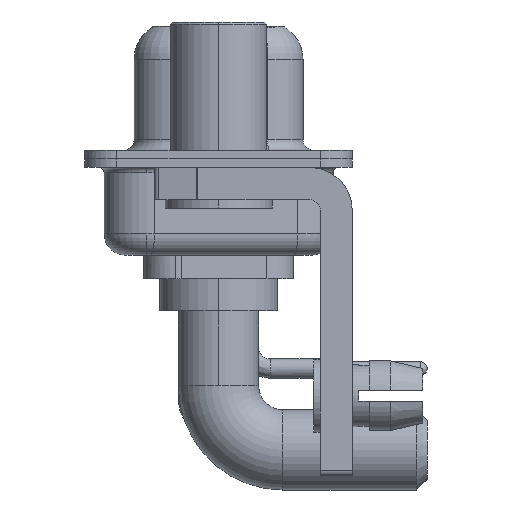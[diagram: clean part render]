
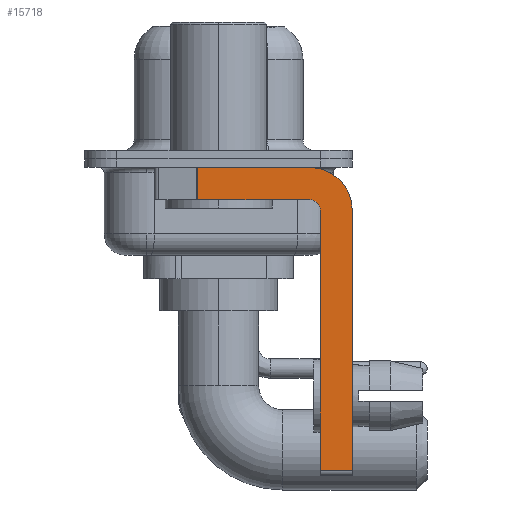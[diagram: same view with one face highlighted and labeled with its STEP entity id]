
A CAD part, left-side view. The second image highlights one B-rep face of the part: STEP entity #15718.
In plain terms, the highlighted planar face has unit normal (-1, 0, 0).
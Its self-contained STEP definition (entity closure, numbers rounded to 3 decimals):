
#17 = ORIENTED_EDGE ( 'NONE', *, *, #8436, .F. ) ;
#399 = CARTESIAN_POINT ( 'NONE',  ( -2.9, 0.978, -1.9 ) ) ;
#597 = VERTEX_POINT ( 'NONE', #4582 ) ;
#678 = EDGE_CURVE ( 'NONE', #4930, #9148, #13054, .T. ) ;
#1188 = CARTESIAN_POINT ( 'NONE',  ( -2.9, -4.75, -14.55 ) ) ;
#1609 = CARTESIAN_POINT ( 'NONE',  ( -2.9, -4.25, -1.9 ) ) ;
#1646 = CARTESIAN_POINT ( 'NONE',  ( -2.9, -4.25, -2.4 ) ) ;
#2113 = LINE ( 'NONE', #8440, #13359 ) ;
#2677 = CARTESIAN_POINT ( 'NONE',  ( -2.9, -4.75, -14.8 ) ) ;
#2889 = ORIENTED_EDGE ( 'NONE', *, *, #14092, .T. ) ;
#3079 = FACE_OUTER_BOUND ( 'NONE', #19467, .T. ) ;
#3131 = ORIENTED_EDGE ( 'NONE', *, *, #19340, .F. ) ;
#3288 = VERTEX_POINT ( 'NONE', #1609 ) ;
#3504 = EDGE_CURVE ( 'NONE', #13564, #3627, #6079, .T. ) ;
#3627 = VERTEX_POINT ( 'NONE', #12449 ) ;
#3746 = AXIS2_PLACEMENT_3D ( 'NONE', #14241, #12507, #4745 ) ;
#3774 = AXIS2_PLACEMENT_3D ( 'NONE', #7189, #13382, #18751 ) ;
#3878 = EDGE_CURVE ( 'NONE', #7032, #13564, #2113, .T. ) ;
#3907 = VERTEX_POINT ( 'NONE', #13589 ) ;
#4548 = PLANE ( 'NONE',  #3746 ) ;
#4582 = CARTESIAN_POINT ( 'NONE',  ( -2.9, -4.75, -2.4 ) ) ;
#4745 = DIRECTION ( 'NONE',  ( 0., 0., -1. ) ) ;
#4930 = VERTEX_POINT ( 'NONE', #1188 ) ;
#5859 = CARTESIAN_POINT ( 'NONE',  ( -2.9, -6.25, -14.55 ) ) ;
#6079 = CIRCLE ( 'NONE', #3774, 2. ) ;
#6417 = DIRECTION ( 'NONE',  ( -1., 0., 0. ) ) ;
#6892 = EDGE_CURVE ( 'NONE', #4930, #597, #10350, .T. ) ;
#7032 = VERTEX_POINT ( 'NONE', #11185 ) ;
#7189 = CARTESIAN_POINT ( 'NONE',  ( -2.9, -4.25, -2.4 ) ) ;
#7872 = EDGE_CURVE ( 'NONE', #3627, #9148, #12156, .T. ) ;
#8357 = LINE ( 'NONE', #399, #18548 ) ;
#8436 = EDGE_CURVE ( 'NONE', #597, #3288, #13116, .T. ) ;
#8440 = CARTESIAN_POINT ( 'NONE',  ( -2.9, 3., -0.4 ) ) ;
#9043 = ORIENTED_EDGE ( 'NONE', *, *, #3878, .F. ) ;
#9148 = VERTEX_POINT ( 'NONE', #5859 ) ;
#9483 = ORIENTED_EDGE ( 'NONE', *, *, #678, .T. ) ;
#10350 = LINE ( 'NONE', #2677, #20332 ) ;
#11185 = CARTESIAN_POINT ( 'NONE',  ( -2.9, 0.978, -0.4 ) ) ;
#11782 = VECTOR ( 'NONE', #18347, 1000. ) ;
#12050 = CARTESIAN_POINT ( 'NONE',  ( -2.9, -4.25, -1.9 ) ) ;
#12125 = AXIS2_PLACEMENT_3D ( 'NONE', #1646, #6417, #12823 ) ;
#12156 = LINE ( 'NONE', #17004, #11782 ) ;
#12449 = CARTESIAN_POINT ( 'NONE',  ( -2.9, -6.25, -2.4 ) ) ;
#12507 = DIRECTION ( 'NONE',  ( 1., 0., 0. ) ) ;
#12823 = DIRECTION ( 'NONE',  ( 0., 0., 1. ) ) ;
#13010 = DIRECTION ( 'NONE',  ( 0., 0., -1. ) ) ;
#13054 = LINE ( 'NONE', #17699, #19336 ) ;
#13116 = CIRCLE ( 'NONE', #12125, 0.5 ) ;
#13359 = VECTOR ( 'NONE', #19493, 1000. ) ;
#13382 = DIRECTION ( 'NONE',  ( 1., 0., 0. ) ) ;
#13564 = VERTEX_POINT ( 'NONE', #19137 ) ;
#13589 = CARTESIAN_POINT ( 'NONE',  ( -2.9, 0.978, -1.9 ) ) ;
#14092 = EDGE_CURVE ( 'NONE', #7032, #3907, #8357, .T. ) ;
#14241 = CARTESIAN_POINT ( 'NONE',  ( -2.9, -4.25, -2.4 ) ) ;
#15228 = ORIENTED_EDGE ( 'NONE', *, *, #6892, .F. ) ;
#15690 = VECTOR ( 'NONE', #16690, 1000. ) ;
#15718 = ADVANCED_FACE ( 'NONE', ( #3079 ), #4548, .F. ) ;
#16245 = DIRECTION ( 'NONE',  ( 0., -1., 0. ) ) ;
#16690 = DIRECTION ( 'NONE',  ( 0., 1., 0. ) ) ;
#17004 = CARTESIAN_POINT ( 'NONE',  ( -2.9, -6.25, -2.4 ) ) ;
#17699 = CARTESIAN_POINT ( 'NONE',  ( -2.9, -4.25, -14.55 ) ) ;
#18101 = ORIENTED_EDGE ( 'NONE', *, *, #7872, .F. ) ;
#18297 = DIRECTION ( 'NONE',  ( 0., 0., 1. ) ) ;
#18347 = DIRECTION ( 'NONE',  ( 0., 0., -1. ) ) ;
#18453 = LINE ( 'NONE', #12050, #15690 ) ;
#18548 = VECTOR ( 'NONE', #13010, 1000. ) ;
#18751 = DIRECTION ( 'NONE',  ( 0., 0., -1. ) ) ;
#19137 = CARTESIAN_POINT ( 'NONE',  ( -2.9, -4.25, -0.4 ) ) ;
#19139 = ORIENTED_EDGE ( 'NONE', *, *, #3504, .F. ) ;
#19336 = VECTOR ( 'NONE', #16245, 1000. ) ;
#19340 = EDGE_CURVE ( 'NONE', #3288, #3907, #18453, .T. ) ;
#19467 = EDGE_LOOP ( 'NONE', ( #9043, #2889, #3131, #17, #15228, #9483, #18101, #19139 ) ) ;
#19493 = DIRECTION ( 'NONE',  ( 0., -1., 0. ) ) ;
#20332 = VECTOR ( 'NONE', #18297, 1000. ) ;
